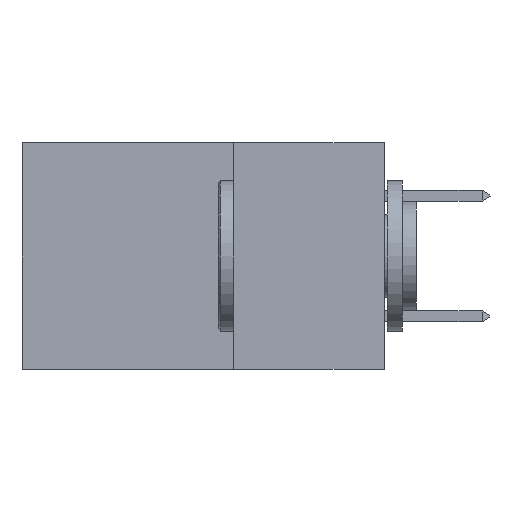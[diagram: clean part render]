
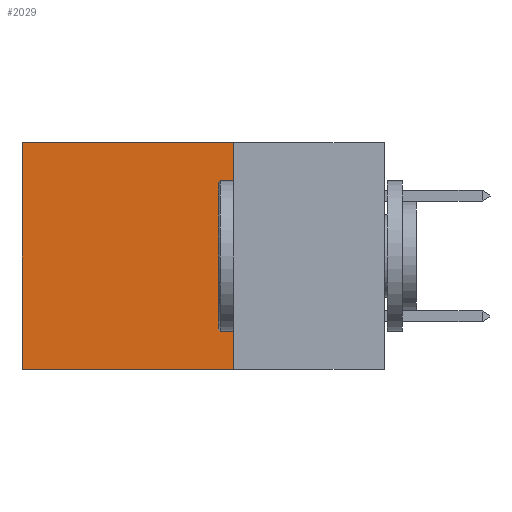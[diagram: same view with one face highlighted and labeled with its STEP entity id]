
A CAD part, left-side view. The second image highlights one B-rep face of the part: STEP entity #2029.
In plain terms, the highlighted planar face has unit normal (-1, 0, 0).
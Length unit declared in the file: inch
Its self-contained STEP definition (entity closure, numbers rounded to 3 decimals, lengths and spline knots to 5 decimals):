
#176 = VERTEX_POINT ( 'NONE', #8650 ) ;
#241 = DIRECTION ( 'NONE',  ( 0., 0., -1. ) ) ;
#394 = CARTESIAN_POINT ( 'NONE',  ( 0.2875, 0.6, -0.375 ) ) ;
#712 = CARTESIAN_POINT ( 'NONE',  ( 0.2875, 0.6, 0. ) ) ;
#740 = LINE ( 'NONE', #394, #8180 ) ;
#860 = LINE ( 'NONE', #5538, #7517 ) ;
#940 = CARTESIAN_POINT ( 'NONE',  ( 0.2875, 0.25, 0. ) ) ;
#985 = LINE ( 'NONE', #4659, #5040 ) ;
#1048 = EDGE_LOOP ( 'NONE', ( #2923, #2799, #1113, #3619 ) ) ;
#1113 = ORIENTED_EDGE ( 'NONE', *, *, #1242, .F. ) ;
#1237 = VECTOR ( 'NONE', #241, 39.37008 ) ;
#1242 = EDGE_CURVE ( 'NONE', #3453, #5387, #8445, .T. ) ;
#1918 = EDGE_CURVE ( 'NONE', #5387, #176, #985, .T. ) ;
#2029 = ADVANCED_FACE ( 'NONE', ( #6724 ), #5560, .F. ) ;
#2410 = AXIS2_PLACEMENT_3D ( 'NONE', #5536, #4050, #6251 ) ;
#2729 = EDGE_CURVE ( 'NONE', #3453, #5744, #860, .T. ) ;
#2748 = DIRECTION ( 'NONE',  ( 0., 1., 0. ) ) ;
#2799 = ORIENTED_EDGE ( 'NONE', *, *, #1918, .F. ) ;
#2923 = ORIENTED_EDGE ( 'NONE', *, *, #8270, .T. ) ;
#3453 = VERTEX_POINT ( 'NONE', #940 ) ;
#3619 = ORIENTED_EDGE ( 'NONE', *, *, #2729, .T. ) ;
#4050 = DIRECTION ( 'NONE',  ( 1., 0., 0. ) ) ;
#4659 = CARTESIAN_POINT ( 'NONE',  ( 0.2875, 0.25, -0.375 ) ) ;
#5040 = VECTOR ( 'NONE', #7471, 39.37008 ) ;
#5267 = CARTESIAN_POINT ( 'NONE',  ( 0.2875, 0.25, -0.375 ) ) ;
#5387 = VERTEX_POINT ( 'NONE', #5997 ) ;
#5536 = CARTESIAN_POINT ( 'NONE',  ( 0.2875, 0.25, -0.375 ) ) ;
#5538 = CARTESIAN_POINT ( 'NONE',  ( 0.2875, 0.25, 0. ) ) ;
#5560 = PLANE ( 'NONE',  #2410 ) ;
#5744 = VERTEX_POINT ( 'NONE', #712 ) ;
#5997 = CARTESIAN_POINT ( 'NONE',  ( 0.2875, 0.25, -0.375 ) ) ;
#6251 = DIRECTION ( 'NONE',  ( 0., 0., -1. ) ) ;
#6724 = FACE_OUTER_BOUND ( 'NONE', #1048, .T. ) ;
#7471 = DIRECTION ( 'NONE',  ( 0., 1., 0. ) ) ;
#7476 = DIRECTION ( 'NONE',  ( 0., 0., -1. ) ) ;
#7517 = VECTOR ( 'NONE', #2748, 39.37008 ) ;
#8180 = VECTOR ( 'NONE', #7476, 39.37008 ) ;
#8270 = EDGE_CURVE ( 'NONE', #5744, #176, #740, .T. ) ;
#8445 = LINE ( 'NONE', #5267, #1237 ) ;
#8650 = CARTESIAN_POINT ( 'NONE',  ( 0.2875, 0.6, -0.375 ) ) ;
